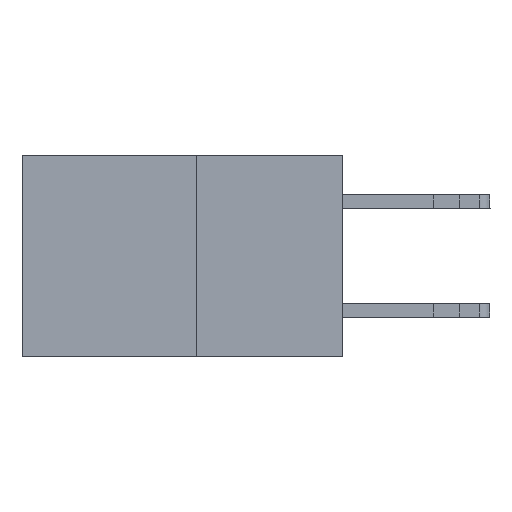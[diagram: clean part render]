
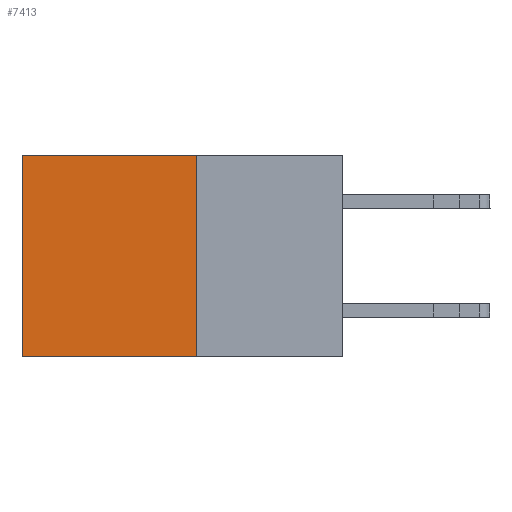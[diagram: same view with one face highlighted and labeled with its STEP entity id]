
A CAD part, left-side view. The second image highlights one B-rep face of the part: STEP entity #7413.
In plain terms, the highlighted planar face has unit normal (-1, 0, 0).
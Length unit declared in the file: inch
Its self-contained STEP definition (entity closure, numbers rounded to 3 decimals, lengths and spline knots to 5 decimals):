
#139 = VECTOR ( 'NONE', #2548, 39.37008 ) ;
#204 = ORIENTED_EDGE ( 'NONE', *, *, #5404, .T. ) ;
#225 = CARTESIAN_POINT ( 'NONE',  ( 0.277, 0.59, 0. ) ) ;
#931 = ORIENTED_EDGE ( 'NONE', *, *, #4155, .F. ) ;
#943 = FACE_OUTER_BOUND ( 'NONE', #12345, .T. ) ;
#1256 = LINE ( 'NONE', #13130, #16266 ) ;
#1422 = CARTESIAN_POINT ( 'NONE',  ( 0.277, 0.27, 0. ) ) ;
#2548 = DIRECTION ( 'NONE',  ( 0., 0., -1. ) ) ;
#2632 = EDGE_CURVE ( 'NONE', #9818, #3257, #7622, .T. ) ;
#2705 = CARTESIAN_POINT ( 'NONE',  ( 0.277, 0.27, -0.37 ) ) ;
#3257 = VERTEX_POINT ( 'NONE', #225 ) ;
#3285 = DIRECTION ( 'NONE',  ( 0., 0., -1. ) ) ;
#3825 = EDGE_CURVE ( 'NONE', #9818, #14553, #4615, .T. ) ;
#4155 = EDGE_CURVE ( 'NONE', #14553, #6216, #14566, .T. ) ;
#4156 = VECTOR ( 'NONE', #5894, 39.37008 ) ;
#4402 = DIRECTION ( 'NONE',  ( 0., 1., 0. ) ) ;
#4429 = CARTESIAN_POINT ( 'NONE',  ( 0.277, 0.27, -0.37 ) ) ;
#4615 = LINE ( 'NONE', #2705, #139 ) ;
#5404 = EDGE_CURVE ( 'NONE', #3257, #6216, #1256, .T. ) ;
#5894 = DIRECTION ( 'NONE',  ( 0., 1., 0. ) ) ;
#6216 = VERTEX_POINT ( 'NONE', #13556 ) ;
#6347 = CARTESIAN_POINT ( 'NONE',  ( 0.277, 0.27, -0.37 ) ) ;
#6966 = CARTESIAN_POINT ( 'NONE',  ( 0.277, 0.27, 0. ) ) ;
#7255 = ORIENTED_EDGE ( 'NONE', *, *, #2632, .T. ) ;
#7413 = ADVANCED_FACE ( 'NONE', ( #943 ), #9157, .F. ) ;
#7622 = LINE ( 'NONE', #1422, #4156 ) ;
#9157 = PLANE ( 'NONE',  #9220 ) ;
#9220 = AXIS2_PLACEMENT_3D ( 'NONE', #10608, #12014, #3285 ) ;
#9818 = VERTEX_POINT ( 'NONE', #6966 ) ;
#10371 = ORIENTED_EDGE ( 'NONE', *, *, #3825, .F. ) ;
#10608 = CARTESIAN_POINT ( 'NONE',  ( 0.277, 0.27, -0.37 ) ) ;
#12014 = DIRECTION ( 'NONE',  ( 1., 0., 0. ) ) ;
#12345 = EDGE_LOOP ( 'NONE', ( #204, #931, #10371, #7255 ) ) ;
#13130 = CARTESIAN_POINT ( 'NONE',  ( 0.277, 0.59, -0.37 ) ) ;
#13556 = CARTESIAN_POINT ( 'NONE',  ( 0.277, 0.59, -0.37 ) ) ;
#14132 = VECTOR ( 'NONE', #4402, 39.37008 ) ;
#14553 = VERTEX_POINT ( 'NONE', #6347 ) ;
#14566 = LINE ( 'NONE', #4429, #14132 ) ;
#15983 = DIRECTION ( 'NONE',  ( 0., 0., -1. ) ) ;
#16266 = VECTOR ( 'NONE', #15983, 39.37008 ) ;
